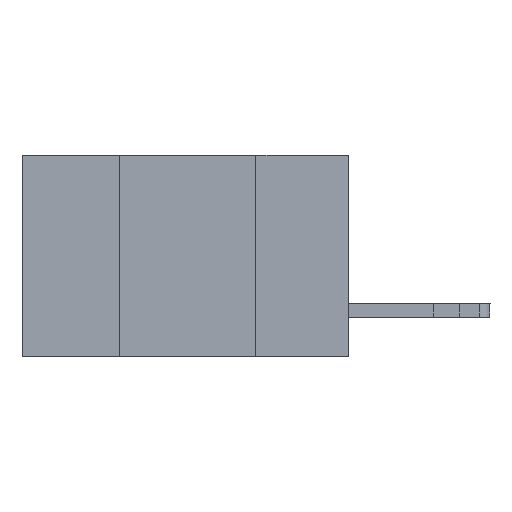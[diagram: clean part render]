
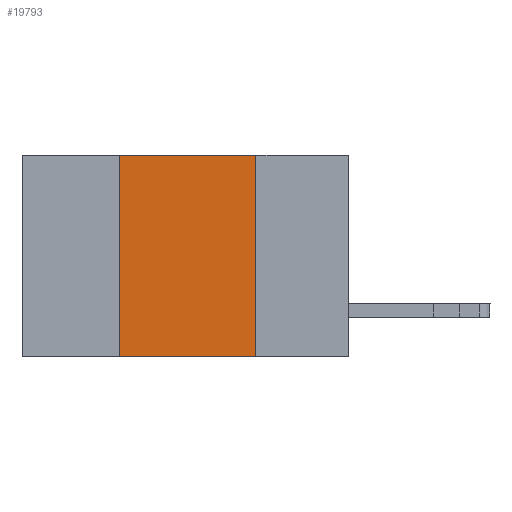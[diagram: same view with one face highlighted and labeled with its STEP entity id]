
A CAD part, left-side view. The second image highlights one B-rep face of the part: STEP entity #19793.
In plain terms, the highlighted planar face has unit normal (-1, 0, 0).
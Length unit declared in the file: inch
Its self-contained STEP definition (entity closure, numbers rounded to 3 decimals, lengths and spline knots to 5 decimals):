
#155 = DIRECTION ( 'NONE',  ( 0., 0., -1. ) ) ;
#810 = EDGE_CURVE ( 'NONE', #10801, #13299, #19231, .T. ) ;
#1372 = LINE ( 'NONE', #22553, #9438 ) ;
#2654 = DIRECTION ( 'NONE',  ( 0., -1., 0. ) ) ;
#2814 = CARTESIAN_POINT ( 'NONE',  ( 0., 0.42, -0.37 ) ) ;
#3990 = CARTESIAN_POINT ( 'NONE',  ( 0., 0.42, 0. ) ) ;
#4413 = CARTESIAN_POINT ( 'NONE',  ( 0., 0.6, 0. ) ) ;
#5219 = EDGE_CURVE ( 'NONE', #19263, #13299, #1372, .T. ) ;
#5883 = VECTOR ( 'NONE', #155, 39.37008 ) ;
#6111 = VECTOR ( 'NONE', #25586, 39.37008 ) ;
#7337 = ORIENTED_EDGE ( 'NONE', *, *, #5219, .T. ) ;
#8042 = EDGE_CURVE ( 'NONE', #19263, #15034, #21345, .T. ) ;
#8326 = DIRECTION ( 'NONE',  ( 0., -1., 0. ) ) ;
#9438 = VECTOR ( 'NONE', #2654, 39.37008 ) ;
#9522 = FACE_OUTER_BOUND ( 'NONE', #13317, .T. ) ;
#10510 = CARTESIAN_POINT ( 'NONE',  ( 0., 0.42, 0. ) ) ;
#10801 = VERTEX_POINT ( 'NONE', #17175 ) ;
#11179 = LINE ( 'NONE', #12473, #18030 ) ;
#12473 = CARTESIAN_POINT ( 'NONE',  ( 0., 0.6, 0. ) ) ;
#12474 = DIRECTION ( 'NONE',  ( 0., 0., -1. ) ) ;
#12583 = ORIENTED_EDGE ( 'NONE', *, *, #810, .F. ) ;
#13299 = VERTEX_POINT ( 'NONE', #18166 ) ;
#13317 = EDGE_LOOP ( 'NONE', ( #12583, #21360, #21750, #7337 ) ) ;
#14743 = AXIS2_PLACEMENT_3D ( 'NONE', #4413, #20377, #12474 ) ;
#15034 = VERTEX_POINT ( 'NONE', #10510 ) ;
#17175 = CARTESIAN_POINT ( 'NONE',  ( 0., 0.17, 0. ) ) ;
#17779 = EDGE_CURVE ( 'NONE', #15034, #10801, #11179, .T. ) ;
#17913 = CARTESIAN_POINT ( 'NONE',  ( 0., 0.17, 0. ) ) ;
#18030 = VECTOR ( 'NONE', #8326, 39.37008 ) ;
#18166 = CARTESIAN_POINT ( 'NONE',  ( 0., 0.17, -0.37 ) ) ;
#18481 = PLANE ( 'NONE',  #14743 ) ;
#19231 = LINE ( 'NONE', #17913, #5883 ) ;
#19263 = VERTEX_POINT ( 'NONE', #2814 ) ;
#19793 = ADVANCED_FACE ( 'NONE', ( #9522 ), #18481, .F. ) ;
#20377 = DIRECTION ( 'NONE',  ( 1., 0., 0. ) ) ;
#21345 = LINE ( 'NONE', #3990, #6111 ) ;
#21360 = ORIENTED_EDGE ( 'NONE', *, *, #17779, .F. ) ;
#21750 = ORIENTED_EDGE ( 'NONE', *, *, #8042, .F. ) ;
#22553 = CARTESIAN_POINT ( 'NONE',  ( 0., 0.6, -0.37 ) ) ;
#25586 = DIRECTION ( 'NONE',  ( 0., 0., 1. ) ) ;
